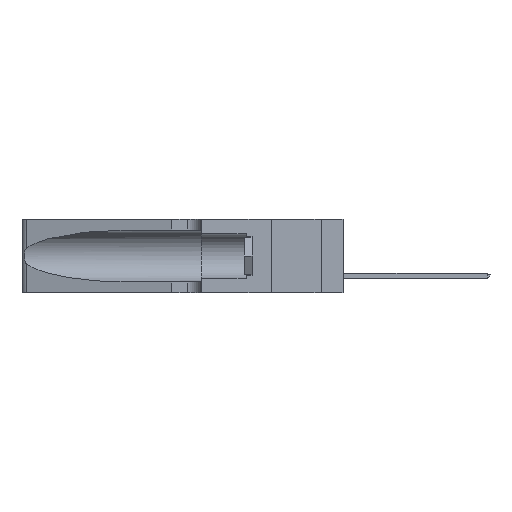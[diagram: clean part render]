
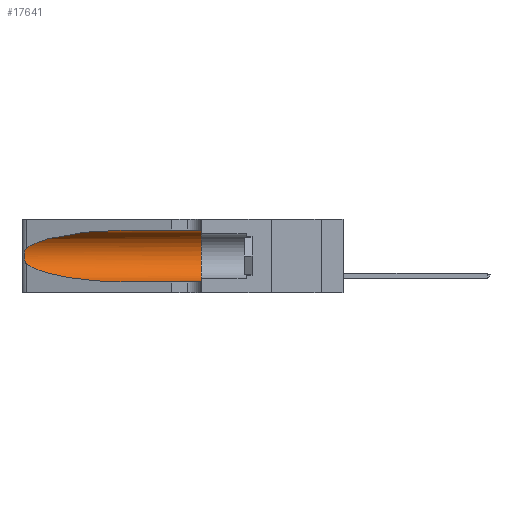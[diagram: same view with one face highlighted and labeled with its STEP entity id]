
A CAD part, left-side view. The second image highlights one B-rep face of the part: STEP entity #17641.
In plain terms, the highlighted cylindrical face has radius 3.308 mm (diameter 6.617 mm), a partial arc.
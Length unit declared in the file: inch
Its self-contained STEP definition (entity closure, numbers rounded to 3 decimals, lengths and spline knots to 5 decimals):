
#159 = CARTESIAN_POINT ( 'NONE',  ( 0.25555, 1.22994, 0.2215 ) ) ;
#397 = CARTESIAN_POINT ( 'NONE',  ( 0.26017, 1.23833, 0.17102 ) ) ;
#496 = EDGE_CURVE ( 'NONE', #3051, #5224, #14611, .T. ) ;
#1478 = LINE ( 'NONE', #11556, #8631 ) ;
#1504 = CARTESIAN_POINT ( 'NONE',  ( 0.1305, 0.35, 0.05475 ) ) ;
#1693 = CARTESIAN_POINT ( 'NONE',  ( 0.2373, 1.15595, 0.28018 ) ) ;
#2266 = B_SPLINE_CURVE_WITH_KNOTS ( 'NONE', 3,
 ( #12702, #159, #19446, #9070, #8925, #19600, #10901, #21134, #397, #7126, #12410, #12627, #3793, #9225 ),
 .UNSPECIFIED., .F., .F.,
 ( 4, 2, 2, 2, 2, 2, 4 ),
 ( 0., 0.00027, 0.00053, 0.00107, 0.0016, 0.00187, 0.00214 ),
 .UNSPECIFIED. ) ;
#2707 = CARTESIAN_POINT ( 'NONE',  ( 0.25487, 1.22718, 0.14631 ) ) ;
#3051 = VERTEX_POINT ( 'NONE', #12447 ) ;
#3568 = VECTOR ( 'NONE', #14572, 39.37008 ) ;
#3742 = CARTESIAN_POINT ( 'NONE',  ( 0.1305, 0.35, 0.185 ) ) ;
#3793 = CARTESIAN_POINT ( 'NONE',  ( 0.25555, 1.22993, 0.14849 ) ) ;
#4466 = ORIENTED_EDGE ( 'NONE', *, *, #12263, .T. ) ;
#4988 = CARTESIAN_POINT ( 'NONE',  ( 0.25487, 1.22718, 0.22369 ) ) ;
#5028 = ORIENTED_EDGE ( 'NONE', *, *, #16601, .T. ) ;
#5204 = EDGE_LOOP ( 'NONE', ( #5695, #18747, #5028, #4466, #11480, #19803 ) ) ;
#5224 = VERTEX_POINT ( 'NONE', #12106 ) ;
#5657 = CARTESIAN_POINT ( 'NONE',  ( 0.1305, 1.61858, 0.31525 ) ) ;
#5695 = ORIENTED_EDGE ( 'NONE', *, *, #496, .T. ) ;
#6920 = CARTESIAN_POINT ( 'NONE',  ( 0.1305, 0.72297, 0.31525 ) ) ;
#7055 = CIRCLE ( 'NONE', #18578, 0.13025 ) ;
#7126 = CARTESIAN_POINT ( 'NONE',  ( 0.25856, 1.23593, 0.16098 ) ) ;
#7627 = VERTEX_POINT ( 'NONE', #12284 ) ;
#7660 = LINE ( 'NONE', #5657, #3568 ) ;
#7672 = DIRECTION ( 'NONE',  ( 0., -1., 0. ) ) ;
#7839 = CARTESIAN_POINT ( 'NONE',  ( 0.1305, 1.61858, 0.185 ) ) ;
#8130 = EDGE_CURVE ( 'NONE', #5224, #7627, #2266, .T. ) ;
#8373 = CARTESIAN_POINT ( 'NONE',  ( 0.2373, 1.15595, 0.08982 ) ) ;
#8631 = VECTOR ( 'NONE', #13284, 39.37008 ) ;
#8925 = CARTESIAN_POINT ( 'NONE',  ( 0.25854, 1.2359, 0.20912 ) ) ;
#8989 = CARTESIAN_POINT ( 'NONE',  ( 0.1305, 0.72297, 0.05475 ) ) ;
#8997 = FACE_OUTER_BOUND ( 'NONE', #5204, .T. ) ;
#9070 = CARTESIAN_POINT ( 'NONE',  ( 0.25787, 1.23484, 0.2124 ) ) ;
#9225 = CARTESIAN_POINT ( 'NONE',  ( 0.25487, 1.22718, 0.14631 ) ) ;
#9606 = EDGE_CURVE ( 'NONE', #18883, #13681, #7055, .T. ) ;
#10701 = DIRECTION ( 'NONE',  ( 0., 1., 0. ) ) ;
#10901 = CARTESIAN_POINT ( 'NONE',  ( 0.26075, 1.23896, 0.19203 ) ) ;
#11480 = ORIENTED_EDGE ( 'NONE', *, *, #9606, .F. ) ;
#11556 = CARTESIAN_POINT ( 'NONE',  ( 0.1305, 1.61858, 0.05475 ) ) ;
#12106 = CARTESIAN_POINT ( 'NONE',  ( 0.25487, 1.22718, 0.22369 ) ) ;
#12263 = EDGE_CURVE ( 'NONE', #12522, #13681, #1478, .T. ) ;
#12284 = CARTESIAN_POINT ( 'NONE',  ( 0.25487, 1.22718, 0.14631 ) ) ;
#12359 = DIRECTION ( 'NONE',  ( 0., 0., 1. ) ) ;
#12410 = CARTESIAN_POINT ( 'NONE',  ( 0.25789, 1.23486, 0.15765 ) ) ;
#12447 = CARTESIAN_POINT ( 'NONE',  ( 0.1305, 0.72297, 0.31525 ) ) ;
#12522 = VERTEX_POINT ( 'NONE', #20557 ) ;
#12627 = CARTESIAN_POINT ( 'NONE',  ( 0.25639, 1.23186, 0.15144 ) ) ;
#12702 = CARTESIAN_POINT ( 'NONE',  ( 0.25487, 1.22718, 0.22369 ) ) ;
#13284 = DIRECTION ( 'NONE',  ( 0., -1., 0. ) ) ;
#13328 =( BOUNDED_CURVE ( )  B_SPLINE_CURVE ( 3, ( #2707, #8373, #20890, #8989 ),
 .UNSPECIFIED., .F., .T. ) 
 B_SPLINE_CURVE_WITH_KNOTS ( ( 4, 4 ),
 ( 3.44316, 4.71239 ),
 .UNSPECIFIED. ) 
 CURVE ( )  GEOMETRIC_REPRESENTATION_ITEM ( )  RATIONAL_B_SPLINE_CURVE ( ( 1., 0.87, 0.87, 1. ) ) 
 REPRESENTATION_ITEM ( '' )  );
#13681 = VERTEX_POINT ( 'NONE', #1504 ) ;
#14572 = DIRECTION ( 'NONE',  ( 0., -1., 0. ) ) ;
#14611 =( BOUNDED_CURVE ( )  B_SPLINE_CURVE ( 3, ( #6920, #22314, #1693, #4988 ),
 .UNSPECIFIED., .F., .F. ) 
 B_SPLINE_CURVE_WITH_KNOTS ( ( 4, 4 ),
 ( 1.5708, 2.84003 ),
 .UNSPECIFIED. ) 
 CURVE ( )  GEOMETRIC_REPRESENTATION_ITEM ( )  RATIONAL_B_SPLINE_CURVE ( ( 1., 0.87, 0.87, 1. ) ) 
 REPRESENTATION_ITEM ( '' )  );
#16601 = EDGE_CURVE ( 'NONE', #7627, #12522, #13328, .T. ) ;
#17115 = CARTESIAN_POINT ( 'NONE',  ( 0.1305, 0.35, 0.31525 ) ) ;
#17641 = ADVANCED_FACE ( 'NONE', ( #8997 ), #22041, .F. ) ;
#18578 = AXIS2_PLACEMENT_3D ( 'NONE', #3742, #10701, #12359 ) ;
#18747 = ORIENTED_EDGE ( 'NONE', *, *, #8130, .T. ) ;
#18883 = VERTEX_POINT ( 'NONE', #17115 ) ;
#19446 = CARTESIAN_POINT ( 'NONE',  ( 0.25639, 1.23184, 0.21858 ) ) ;
#19600 = CARTESIAN_POINT ( 'NONE',  ( 0.26018, 1.23835, 0.19895 ) ) ;
#19803 = ORIENTED_EDGE ( 'NONE', *, *, #20076, .F. ) ;
#20076 = EDGE_CURVE ( 'NONE', #3051, #18883, #7660, .T. ) ;
#20198 = AXIS2_PLACEMENT_3D ( 'NONE', #7839, #7672, #21593 ) ;
#20557 = CARTESIAN_POINT ( 'NONE',  ( 0.1305, 0.72297, 0.05475 ) ) ;
#20890 = CARTESIAN_POINT ( 'NONE',  ( 0.18966, 0.96281, 0.05475 ) ) ;
#21134 = CARTESIAN_POINT ( 'NONE',  ( 0.26075, 1.23896, 0.178 ) ) ;
#21593 = DIRECTION ( 'NONE',  ( 0., 0., -1. ) ) ;
#22041 = CYLINDRICAL_SURFACE ( 'NONE', #20198, 0.13025 ) ;
#22314 = CARTESIAN_POINT ( 'NONE',  ( 0.18966, 0.96281, 0.31525 ) ) ;
